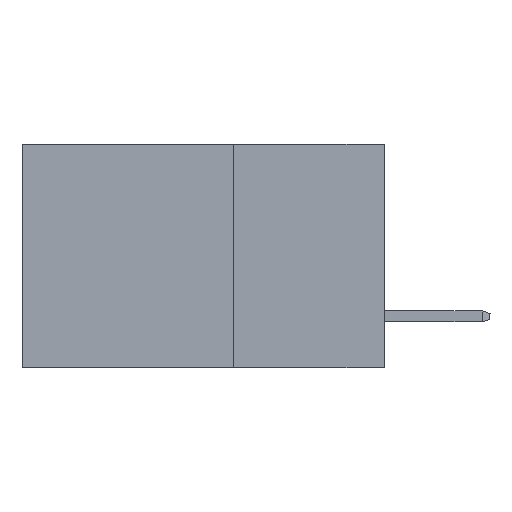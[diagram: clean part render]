
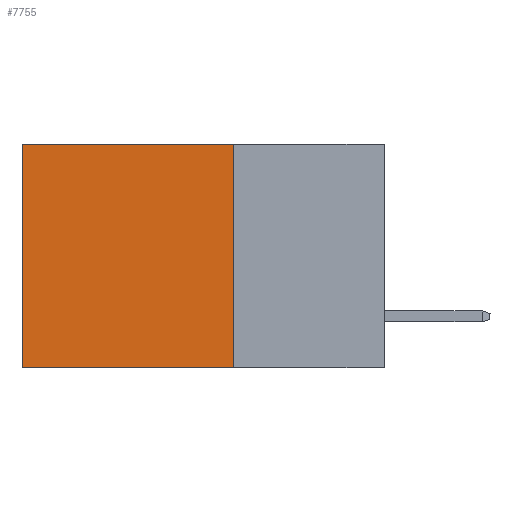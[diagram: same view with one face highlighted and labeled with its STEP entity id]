
A CAD part, left-side view. The second image highlights one B-rep face of the part: STEP entity #7755.
In plain terms, the highlighted planar face has unit normal (-1, 0, 0).
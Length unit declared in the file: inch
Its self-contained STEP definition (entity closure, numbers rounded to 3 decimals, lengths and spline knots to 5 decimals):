
#68 = VECTOR ( 'NONE', #17729, 39.37008 ) ;
#680 = AXIS2_PLACEMENT_3D ( 'NONE', #13839, #1367, #14380 ) ;
#1115 = LINE ( 'NONE', #10882, #1285 ) ;
#1285 = VECTOR ( 'NONE', #4034, 39.37008 ) ;
#1367 = DIRECTION ( 'NONE',  ( 1., 0., 0. ) ) ;
#1727 = ORIENTED_EDGE ( 'NONE', *, *, #13019, .T. ) ;
#2058 = LINE ( 'NONE', #6548, #68 ) ;
#2483 = VERTEX_POINT ( 'NONE', #4828 ) ;
#2599 = LINE ( 'NONE', #13934, #7800 ) ;
#3553 = LINE ( 'NONE', #5062, #5992 ) ;
#3975 = EDGE_CURVE ( 'NONE', #12613, #9198, #3553, .T. ) ;
#3979 = EDGE_LOOP ( 'NONE', ( #13758, #9462, #14217, #1727 ) ) ;
#4034 = DIRECTION ( 'NONE',  ( 0., 0., -1. ) ) ;
#4187 = DIRECTION ( 'NONE',  ( 0., 1., 0. ) ) ;
#4828 = CARTESIAN_POINT ( 'NONE',  ( 0.2615, 0.6, -0.37 ) ) ;
#5062 = CARTESIAN_POINT ( 'NONE',  ( 0.2615, 0.25, -0.37 ) ) ;
#5123 = CARTESIAN_POINT ( 'NONE',  ( 0.2615, 0.25, -0.37 ) ) ;
#5992 = VECTOR ( 'NONE', #10774, 39.37008 ) ;
#6548 = CARTESIAN_POINT ( 'NONE',  ( 0.2615, 0.25, -0.37 ) ) ;
#7755 = ADVANCED_FACE ( 'NONE', ( #12337 ), #18089, .F. ) ;
#7800 = VECTOR ( 'NONE', #4187, 39.37008 ) ;
#9198 = VERTEX_POINT ( 'NONE', #5123 ) ;
#9462 = ORIENTED_EDGE ( 'NONE', *, *, #15222, .F. ) ;
#10774 = DIRECTION ( 'NONE',  ( 0., 0., -1. ) ) ;
#10882 = CARTESIAN_POINT ( 'NONE',  ( 0.2615, 0.6, -0.37 ) ) ;
#12337 = FACE_OUTER_BOUND ( 'NONE', #3979, .T. ) ;
#12613 = VERTEX_POINT ( 'NONE', #17160 ) ;
#13019 = EDGE_CURVE ( 'NONE', #12613, #14807, #2599, .T. ) ;
#13758 = ORIENTED_EDGE ( 'NONE', *, *, #17573, .T. ) ;
#13839 = CARTESIAN_POINT ( 'NONE',  ( 0.2615, 0.25, -0.37 ) ) ;
#13934 = CARTESIAN_POINT ( 'NONE',  ( 0.2615, 0.25, 0. ) ) ;
#14217 = ORIENTED_EDGE ( 'NONE', *, *, #3975, .F. ) ;
#14380 = DIRECTION ( 'NONE',  ( 0., 0., -1. ) ) ;
#14807 = VERTEX_POINT ( 'NONE', #16715 ) ;
#15222 = EDGE_CURVE ( 'NONE', #9198, #2483, #2058, .T. ) ;
#16715 = CARTESIAN_POINT ( 'NONE',  ( 0.2615, 0.6, 0. ) ) ;
#17160 = CARTESIAN_POINT ( 'NONE',  ( 0.2615, 0.25, 0. ) ) ;
#17573 = EDGE_CURVE ( 'NONE', #14807, #2483, #1115, .T. ) ;
#17729 = DIRECTION ( 'NONE',  ( 0., 1., 0. ) ) ;
#18089 = PLANE ( 'NONE',  #680 ) ;
